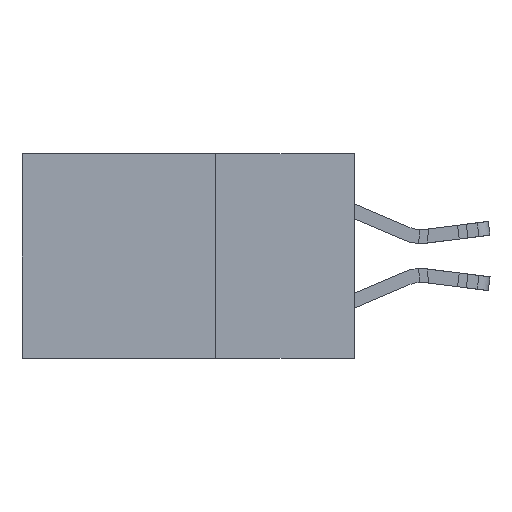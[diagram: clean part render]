
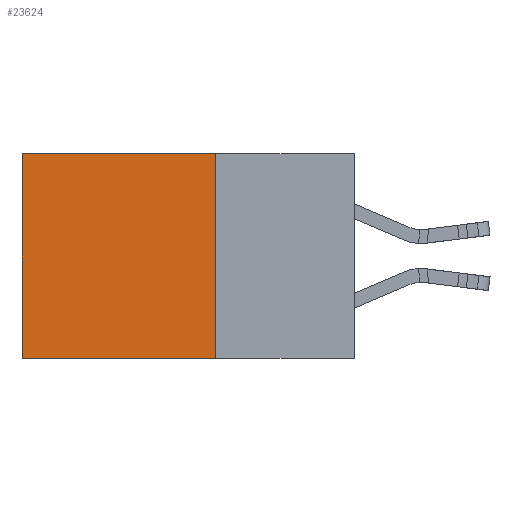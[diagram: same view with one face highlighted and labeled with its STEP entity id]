
A CAD part, left-side view. The second image highlights one B-rep face of the part: STEP entity #23624.
In plain terms, the highlighted planar face has unit normal (-1, 0, 0).
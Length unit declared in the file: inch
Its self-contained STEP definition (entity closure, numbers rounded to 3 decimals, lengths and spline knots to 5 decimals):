
#2381 = CARTESIAN_POINT ( 'NONE',  ( 0.2615, 0.6, 0. ) ) ;
#4785 = EDGE_LOOP ( 'NONE', ( #6544, #11196, #8586, #11382 ) ) ;
#5270 = EDGE_CURVE ( 'NONE', #13306, #9468, #20940, .T. ) ;
#5300 = LINE ( 'NONE', #9635, #15924 ) ;
#5708 = DIRECTION ( 'NONE',  ( 0., 0., -1. ) ) ;
#6544 = ORIENTED_EDGE ( 'NONE', *, *, #10768, .T. ) ;
#6752 = CARTESIAN_POINT ( 'NONE',  ( 0.2615, 0.6, -0.37 ) ) ;
#7916 = CARTESIAN_POINT ( 'NONE',  ( 0.2615, 0.25, -0.37 ) ) ;
#7969 = CARTESIAN_POINT ( 'NONE',  ( 0.2615, 0.25, -0.37 ) ) ;
#8586 = ORIENTED_EDGE ( 'NONE', *, *, #5270, .F. ) ;
#8641 = CARTESIAN_POINT ( 'NONE',  ( 0.2615, 0.25, 0. ) ) ;
#9468 = VERTEX_POINT ( 'NONE', #7916 ) ;
#9635 = CARTESIAN_POINT ( 'NONE',  ( 0.2615, 0.25, 0. ) ) ;
#9655 = VECTOR ( 'NONE', #5708, 39.37008 ) ;
#10768 = EDGE_CURVE ( 'NONE', #12496, #11226, #19675, .T. ) ;
#10786 = AXIS2_PLACEMENT_3D ( 'NONE', #7969, #27062, #14372 ) ;
#11196 = ORIENTED_EDGE ( 'NONE', *, *, #20153, .F. ) ;
#11226 = VERTEX_POINT ( 'NONE', #6752 ) ;
#11382 = ORIENTED_EDGE ( 'NONE', *, *, #27314, .T. ) ;
#11780 = DIRECTION ( 'NONE',  ( 0., 1., 0. ) ) ;
#12162 = PLANE ( 'NONE',  #10786 ) ;
#12496 = VERTEX_POINT ( 'NONE', #2381 ) ;
#13306 = VERTEX_POINT ( 'NONE', #8641 ) ;
#14372 = DIRECTION ( 'NONE',  ( 0., 0., -1. ) ) ;
#14681 = VECTOR ( 'NONE', #15933, 39.37008 ) ;
#15924 = VECTOR ( 'NONE', #11780, 39.37008 ) ;
#15933 = DIRECTION ( 'NONE',  ( 0., 0., -1. ) ) ;
#16016 = FACE_OUTER_BOUND ( 'NONE', #4785, .T. ) ;
#17788 = CARTESIAN_POINT ( 'NONE',  ( 0.2615, 0.25, -0.37 ) ) ;
#19675 = LINE ( 'NONE', #22261, #14681 ) ;
#20153 = EDGE_CURVE ( 'NONE', #9468, #11226, #20237, .T. ) ;
#20237 = LINE ( 'NONE', #17788, #25214 ) ;
#20940 = LINE ( 'NONE', #22703, #9655 ) ;
#22098 = DIRECTION ( 'NONE',  ( 0., 1., 0. ) ) ;
#22261 = CARTESIAN_POINT ( 'NONE',  ( 0.2615, 0.6, -0.37 ) ) ;
#22703 = CARTESIAN_POINT ( 'NONE',  ( 0.2615, 0.25, -0.37 ) ) ;
#23624 = ADVANCED_FACE ( 'NONE', ( #16016 ), #12162, .F. ) ;
#25214 = VECTOR ( 'NONE', #22098, 39.37008 ) ;
#27062 = DIRECTION ( 'NONE',  ( 1., 0., 0. ) ) ;
#27314 = EDGE_CURVE ( 'NONE', #13306, #12496, #5300, .T. ) ;
